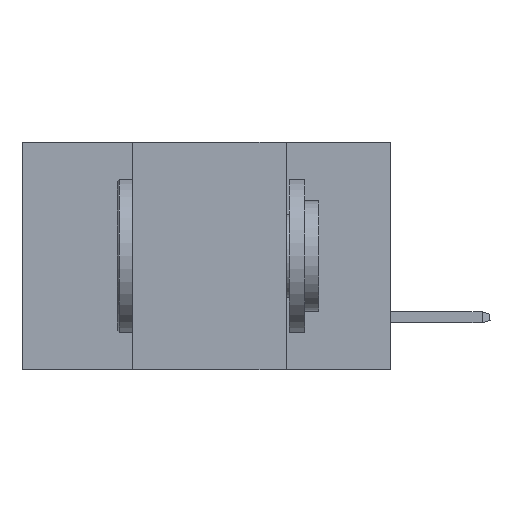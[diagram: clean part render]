
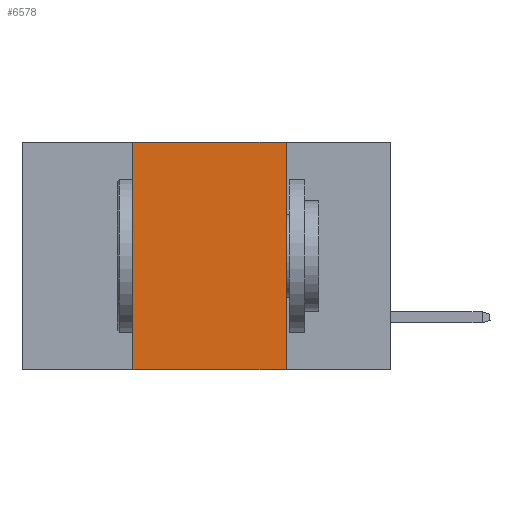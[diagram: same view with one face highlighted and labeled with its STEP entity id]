
A CAD part, left-side view. The second image highlights one B-rep face of the part: STEP entity #6578.
In plain terms, the highlighted planar face has unit normal (-1, 0, 0).
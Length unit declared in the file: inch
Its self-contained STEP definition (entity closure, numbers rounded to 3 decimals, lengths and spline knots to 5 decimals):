
#46 = CARTESIAN_POINT ( 'NONE',  ( 0., 0.17, -0.37 ) ) ;
#2698 = VERTEX_POINT ( 'NONE', #27930 ) ;
#4225 = ORIENTED_EDGE ( 'NONE', *, *, #30611, .F. ) ;
#4927 = VERTEX_POINT ( 'NONE', #9868 ) ;
#5984 = EDGE_CURVE ( 'NONE', #4927, #10047, #14360, .T. ) ;
#6578 = ADVANCED_FACE ( 'NONE', ( #35358 ), #28928, .F. ) ;
#9544 = CARTESIAN_POINT ( 'NONE',  ( 0., 0.6, 0. ) ) ;
#9732 = DIRECTION ( 'NONE',  ( 0., 0., -1. ) ) ;
#9868 = CARTESIAN_POINT ( 'NONE',  ( 0., 0.17, 0. ) ) ;
#10047 = VERTEX_POINT ( 'NONE', #46 ) ;
#10067 = VECTOR ( 'NONE', #24800, 39.37008 ) ;
#10441 = CARTESIAN_POINT ( 'NONE',  ( 0., 0.6, -0.37 ) ) ;
#12211 = ORIENTED_EDGE ( 'NONE', *, *, #5984, .F. ) ;
#13042 = LINE ( 'NONE', #10441, #10067 ) ;
#14360 = LINE ( 'NONE', #17897, #31542 ) ;
#14435 = ORIENTED_EDGE ( 'NONE', *, *, #34618, .T. ) ;
#15981 = AXIS2_PLACEMENT_3D ( 'NONE', #18082, #34779, #9732 ) ;
#16118 = VECTOR ( 'NONE', #32861, 39.37008 ) ;
#17238 = LINE ( 'NONE', #9544, #31388 ) ;
#17897 = CARTESIAN_POINT ( 'NONE',  ( 0., 0.17, 0. ) ) ;
#18082 = CARTESIAN_POINT ( 'NONE',  ( 0., 0.6, 0. ) ) ;
#19130 = EDGE_LOOP ( 'NONE', ( #12211, #4225, #21603, #14435 ) ) ;
#21374 = CARTESIAN_POINT ( 'NONE',  ( 0., 0.42, 0. ) ) ;
#21603 = ORIENTED_EDGE ( 'NONE', *, *, #33376, .F. ) ;
#24656 = VERTEX_POINT ( 'NONE', #32063 ) ;
#24800 = DIRECTION ( 'NONE',  ( 0., -1., 0. ) ) ;
#27930 = CARTESIAN_POINT ( 'NONE',  ( 0., 0.42, -0.37 ) ) ;
#28928 = PLANE ( 'NONE',  #15981 ) ;
#29182 = DIRECTION ( 'NONE',  ( 0., 0., -1. ) ) ;
#30611 = EDGE_CURVE ( 'NONE', #24656, #4927, #17238, .T. ) ;
#31169 = LINE ( 'NONE', #21374, #16118 ) ;
#31388 = VECTOR ( 'NONE', #31440, 39.37008 ) ;
#31440 = DIRECTION ( 'NONE',  ( 0., -1., 0. ) ) ;
#31542 = VECTOR ( 'NONE', #29182, 39.37008 ) ;
#32063 = CARTESIAN_POINT ( 'NONE',  ( 0., 0.42, 0. ) ) ;
#32861 = DIRECTION ( 'NONE',  ( 0., 0., 1. ) ) ;
#33376 = EDGE_CURVE ( 'NONE', #2698, #24656, #31169, .T. ) ;
#34618 = EDGE_CURVE ( 'NONE', #2698, #10047, #13042, .T. ) ;
#34779 = DIRECTION ( 'NONE',  ( 1., 0., 0. ) ) ;
#35358 = FACE_OUTER_BOUND ( 'NONE', #19130, .T. ) ;
